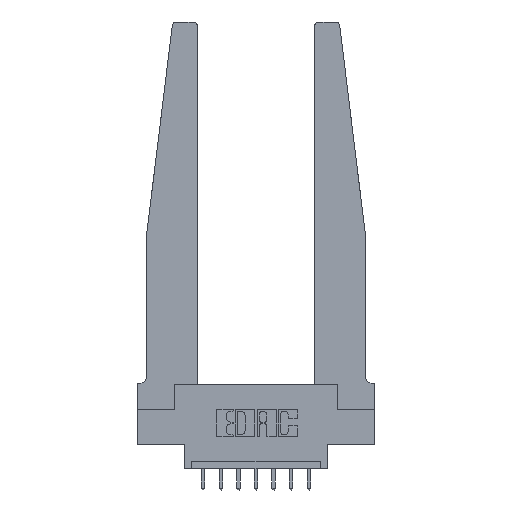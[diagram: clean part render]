
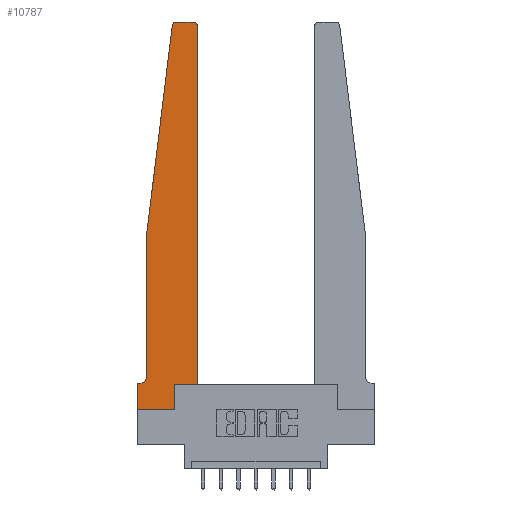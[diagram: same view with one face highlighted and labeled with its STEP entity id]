
A CAD part, top view. The second image highlights one B-rep face of the part: STEP entity #10787.
In plain terms, the highlighted planar face has unit normal (0, 0, 1).
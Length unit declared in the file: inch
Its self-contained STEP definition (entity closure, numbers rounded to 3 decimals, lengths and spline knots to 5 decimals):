
#80 = AXIS2_PLACEMENT_3D ( 'NONE', #2588, #4874, #4721 ) ;
#82 = DIRECTION ( 'NONE',  ( 0., 0., 1. ) ) ;
#113 = EDGE_CURVE ( 'NONE', #133, #13842, #235, .T. ) ;
#133 = VERTEX_POINT ( 'NONE', #5638 ) ;
#142 = CARTESIAN_POINT ( 'NONE',  ( 0.065, 0.1875, 0.37 ) ) ;
#235 = CIRCLE ( 'NONE', #10957, 0.03 ) ;
#311 = VERTEX_POINT ( 'NONE', #373 ) ;
#331 = EDGE_CURVE ( 'NONE', #5494, #11227, #507, .T. ) ;
#373 = CARTESIAN_POINT ( 'NONE',  ( 0.395, 2.75, 0.37 ) ) ;
#507 = LINE ( 'NONE', #9348, #12599 ) ;
#749 = VERTEX_POINT ( 'NONE', #10029 ) ;
#857 = ORIENTED_EDGE ( 'NONE', *, *, #1224, .T. ) ;
#925 = VERTEX_POINT ( 'NONE', #12513 ) ;
#934 = ORIENTED_EDGE ( 'NONE', *, *, #331, .T. ) ;
#1224 = EDGE_CURVE ( 'NONE', #11227, #749, #13790, .T. ) ;
#1389 = CARTESIAN_POINT ( 'NONE',  ( 0.425, 0.18, 0.37 ) ) ;
#1430 = ORIENTED_EDGE ( 'NONE', *, *, #3599, .T. ) ;
#1526 = ORIENTED_EDGE ( 'NONE', *, *, #10942, .T. ) ;
#1784 = ORIENTED_EDGE ( 'NONE', *, *, #4714, .T. ) ;
#2464 = VERTEX_POINT ( 'NONE', #4784 ) ;
#2588 = CARTESIAN_POINT ( 'NONE',  ( 0.395, 2.72, 0.37 ) ) ;
#2816 = DIRECTION ( 'NONE',  ( 0., 1., 0. ) ) ;
#2876 = DIRECTION ( 'NONE',  ( -0.122, -0.992, 0. ) ) ;
#2957 = VECTOR ( 'NONE', #10111, 39.37008 ) ;
#3066 = DIRECTION ( 'NONE',  ( 0., 0., 1. ) ) ;
#3088 = CIRCLE ( 'NONE', #8197, 0.05 ) ;
#3302 = CARTESIAN_POINT ( 'NONE',  ( 0.27653, 2.72, 0.37 ) ) ;
#3599 = EDGE_CURVE ( 'NONE', #5433, #6351, #9250, .T. ) ;
#3768 = ORIENTED_EDGE ( 'NONE', *, *, #10053, .T. ) ;
#4142 = CARTESIAN_POINT ( 'NONE',  ( 0.2605, 0.18, 0.37 ) ) ;
#4276 = EDGE_CURVE ( 'NONE', #13842, #925, #8341, .T. ) ;
#4622 = LINE ( 'NONE', #142, #5662 ) ;
#4714 = EDGE_CURVE ( 'NONE', #2464, #5433, #4936, .T. ) ;
#4721 = DIRECTION ( 'NONE',  ( 1., 0., 0. ) ) ;
#4753 = DIRECTION ( 'NONE',  ( 1., 0., 0. ) ) ;
#4765 = VECTOR ( 'NONE', #8231, 39.37008 ) ;
#4784 = CARTESIAN_POINT ( 'NONE',  ( 0., 0.1875, 0.37 ) ) ;
#4874 = DIRECTION ( 'NONE',  ( 0., 0., 1. ) ) ;
#4936 = LINE ( 'NONE', #9362, #7499 ) ;
#4996 = EDGE_CURVE ( 'NONE', #9573, #12736, #3088, .T. ) ;
#5055 = DIRECTION ( 'NONE',  ( 1., 0., 0. ) ) ;
#5229 = ORIENTED_EDGE ( 'NONE', *, *, #113, .T. ) ;
#5332 = ORIENTED_EDGE ( 'NONE', *, *, #4996, .T. ) ;
#5433 = VERTEX_POINT ( 'NONE', #9527 ) ;
#5494 = VERTEX_POINT ( 'NONE', #4142 ) ;
#5499 = DIRECTION ( 'NONE',  ( -1., 0., 0. ) ) ;
#5638 = CARTESIAN_POINT ( 'NONE',  ( 0.27653, 2.75, 0.37 ) ) ;
#5662 = VECTOR ( 'NONE', #5499, 39.37008 ) ;
#5722 = CARTESIAN_POINT ( 'NONE',  ( 0.425, 0.18, 0.37 ) ) ;
#5873 = EDGE_CURVE ( 'NONE', #749, #311, #11737, .T. ) ;
#6124 = DIRECTION ( 'NONE',  ( 1., 0., 0. ) ) ;
#6337 = EDGE_LOOP ( 'NONE', ( #7467, #5229, #7859, #14028, #5332, #1526, #1784, #1430, #3768, #934, #857, #11586 ) ) ;
#6351 = VERTEX_POINT ( 'NONE', #8388 ) ;
#6585 = CARTESIAN_POINT ( 'NONE',  ( 0.065, 0.2375, 0.37 ) ) ;
#6590 = CARTESIAN_POINT ( 'NONE',  ( 0.065, 1.25, 0.37 ) ) ;
#6975 = LINE ( 'NONE', #10187, #2957 ) ;
#7379 = CARTESIAN_POINT ( 'NONE',  ( 0., 0.1875, 0.37 ) ) ;
#7467 = ORIENTED_EDGE ( 'NONE', *, *, #13681, .T. ) ;
#7499 = VECTOR ( 'NONE', #13804, 39.37008 ) ;
#7659 = DIRECTION ( 'NONE',  ( 1., 0., 0. ) ) ;
#7859 = ORIENTED_EDGE ( 'NONE', *, *, #4276, .T. ) ;
#7981 = AXIS2_PLACEMENT_3D ( 'NONE', #7379, #3066, #5055 ) ;
#8197 = AXIS2_PLACEMENT_3D ( 'NONE', #9062, #13497, #9201 ) ;
#8231 = DIRECTION ( 'NONE',  ( 0., 1., 0. ) ) ;
#8341 = LINE ( 'NONE', #12809, #12686 ) ;
#8352 = LINE ( 'NONE', #12817, #14015 ) ;
#8388 = CARTESIAN_POINT ( 'NONE',  ( 0.2605, 0., 0.37 ) ) ;
#8716 = LINE ( 'NONE', #6590, #11137 ) ;
#9062 = CARTESIAN_POINT ( 'NONE',  ( 0.015, 0.2375, 0.37 ) ) ;
#9201 = DIRECTION ( 'NONE',  ( -1., 0., 0. ) ) ;
#9250 = LINE ( 'NONE', #13539, #13174 ) ;
#9348 = CARTESIAN_POINT ( 'NONE',  ( 0.425, 0.18, 0.37 ) ) ;
#9362 = CARTESIAN_POINT ( 'NONE',  ( 0., 0., 0.37 ) ) ;
#9527 = CARTESIAN_POINT ( 'NONE',  ( 0., 0., 0.37 ) ) ;
#9573 = VERTEX_POINT ( 'NONE', #6585 ) ;
#9660 = DIRECTION ( 'NONE',  ( 0., -1., 0. ) ) ;
#9708 = PLANE ( 'NONE',  #7981 ) ;
#10029 = CARTESIAN_POINT ( 'NONE',  ( 0.425, 2.72, 0.37 ) ) ;
#10053 = EDGE_CURVE ( 'NONE', #6351, #5494, #8352, .T. ) ;
#10111 = DIRECTION ( 'NONE',  ( -1., 0., 0. ) ) ;
#10187 = CARTESIAN_POINT ( 'NONE',  ( 0.25, 2.75, 0.37 ) ) ;
#10787 = ADVANCED_FACE ( 'NONE', ( #13054 ), #9708, .T. ) ;
#10942 = EDGE_CURVE ( 'NONE', #12736, #2464, #4622, .T. ) ;
#10957 = AXIS2_PLACEMENT_3D ( 'NONE', #3302, #82, #7659 ) ;
#11137 = VECTOR ( 'NONE', #9660, 39.37008 ) ;
#11227 = VERTEX_POINT ( 'NONE', #5722 ) ;
#11586 = ORIENTED_EDGE ( 'NONE', *, *, #5873, .T. ) ;
#11737 = CIRCLE ( 'NONE', #80, 0.03 ) ;
#12513 = CARTESIAN_POINT ( 'NONE',  ( 0.065, 1.25, 0.37 ) ) ;
#12599 = VECTOR ( 'NONE', #6124, 39.37008 ) ;
#12686 = VECTOR ( 'NONE', #2876, 39.37008 ) ;
#12736 = VERTEX_POINT ( 'NONE', #13345 ) ;
#12809 = CARTESIAN_POINT ( 'NONE',  ( 0.065, 1.25, 0.37 ) ) ;
#12817 = CARTESIAN_POINT ( 'NONE',  ( 0.2605, 0.18, 0.37 ) ) ;
#13054 = FACE_OUTER_BOUND ( 'NONE', #6337, .T. ) ;
#13082 = CARTESIAN_POINT ( 'NONE',  ( 0.24675, 2.72367, 0.37 ) ) ;
#13174 = VECTOR ( 'NONE', #4753, 39.37008 ) ;
#13345 = CARTESIAN_POINT ( 'NONE',  ( 0.015, 0.1875, 0.37 ) ) ;
#13497 = DIRECTION ( 'NONE',  ( 0., 0., -1. ) ) ;
#13539 = CARTESIAN_POINT ( 'NONE',  ( 0., 0., 0.37 ) ) ;
#13681 = EDGE_CURVE ( 'NONE', #311, #133, #6975, .T. ) ;
#13790 = LINE ( 'NONE', #1389, #4765 ) ;
#13804 = DIRECTION ( 'NONE',  ( 0., -1., 0. ) ) ;
#13842 = VERTEX_POINT ( 'NONE', #13082 ) ;
#13878 = EDGE_CURVE ( 'NONE', #925, #9573, #8716, .T. ) ;
#14015 = VECTOR ( 'NONE', #2816, 39.37008 ) ;
#14028 = ORIENTED_EDGE ( 'NONE', *, *, #13878, .T. ) ;
